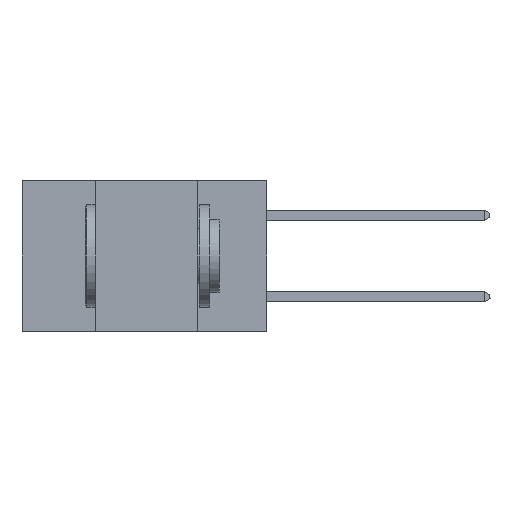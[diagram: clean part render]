
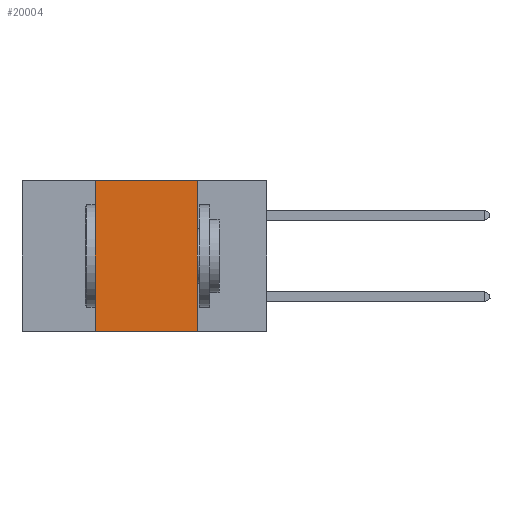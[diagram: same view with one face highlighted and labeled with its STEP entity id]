
A CAD part, left-side view. The second image highlights one B-rep face of the part: STEP entity #20004.
In plain terms, the highlighted planar face has unit normal (-1, 0, 0).
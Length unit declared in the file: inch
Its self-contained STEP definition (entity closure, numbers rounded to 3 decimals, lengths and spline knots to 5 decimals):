
#823 = DIRECTION ( 'NONE',  ( 0., -1., 0. ) ) ;
#4264 = CARTESIAN_POINT ( 'NONE',  ( 0., 0.42, 0. ) ) ;
#5009 = ORIENTED_EDGE ( 'NONE', *, *, #30046, .F. ) ;
#6445 = LINE ( 'NONE', #14325, #34860 ) ;
#6691 = CARTESIAN_POINT ( 'NONE',  ( 0., 0.42, 0. ) ) ;
#8905 = CARTESIAN_POINT ( 'NONE',  ( 0., 0.17, -0.37 ) ) ;
#9382 = DIRECTION ( 'NONE',  ( 0., 0., -1. ) ) ;
#10044 = EDGE_CURVE ( 'NONE', #40471, #34120, #26797, .T. ) ;
#11352 = DIRECTION ( 'NONE',  ( 0., 0., -1. ) ) ;
#12225 = VERTEX_POINT ( 'NONE', #8905 ) ;
#12691 = CARTESIAN_POINT ( 'NONE',  ( 0., 0.42, -0.37 ) ) ;
#14325 = CARTESIAN_POINT ( 'NONE',  ( 0., 0.6, -0.37 ) ) ;
#14375 = DIRECTION ( 'NONE',  ( 0., 0., 1. ) ) ;
#14609 = CARTESIAN_POINT ( 'NONE',  ( 0., 0.6, 0. ) ) ;
#14787 = FACE_OUTER_BOUND ( 'NONE', #19212, .T. ) ;
#15204 = ORIENTED_EDGE ( 'NONE', *, *, #36330, .T. ) ;
#18491 = VERTEX_POINT ( 'NONE', #21373 ) ;
#19212 = EDGE_LOOP ( 'NONE', ( #33640, #5009, #25179, #15204 ) ) ;
#19237 = CARTESIAN_POINT ( 'NONE',  ( 0., 0.6, 0. ) ) ;
#20004 = ADVANCED_FACE ( 'NONE', ( #14787 ), #22216, .F. ) ;
#21175 = EDGE_CURVE ( 'NONE', #18491, #12225, #32630, .T. ) ;
#21373 = CARTESIAN_POINT ( 'NONE',  ( 0., 0.17, 0. ) ) ;
#21675 = DIRECTION ( 'NONE',  ( 0., -1., 0. ) ) ;
#22216 = PLANE ( 'NONE',  #24420 ) ;
#23692 = VECTOR ( 'NONE', #11352, 39.37008 ) ;
#24420 = AXIS2_PLACEMENT_3D ( 'NONE', #19237, #35760, #9382 ) ;
#25179 = ORIENTED_EDGE ( 'NONE', *, *, #10044, .F. ) ;
#26246 = VECTOR ( 'NONE', #14375, 39.37008 ) ;
#26797 = LINE ( 'NONE', #4264, #26246 ) ;
#30046 = EDGE_CURVE ( 'NONE', #34120, #18491, #35390, .T. ) ;
#32630 = LINE ( 'NONE', #38051, #23692 ) ;
#33640 = ORIENTED_EDGE ( 'NONE', *, *, #21175, .F. ) ;
#34120 = VERTEX_POINT ( 'NONE', #6691 ) ;
#34860 = VECTOR ( 'NONE', #823, 39.37008 ) ;
#35390 = LINE ( 'NONE', #14609, #36475 ) ;
#35760 = DIRECTION ( 'NONE',  ( 1., 0., 0. ) ) ;
#36330 = EDGE_CURVE ( 'NONE', #40471, #12225, #6445, .T. ) ;
#36475 = VECTOR ( 'NONE', #21675, 39.37008 ) ;
#38051 = CARTESIAN_POINT ( 'NONE',  ( 0., 0.17, 0. ) ) ;
#40471 = VERTEX_POINT ( 'NONE', #12691 ) ;
